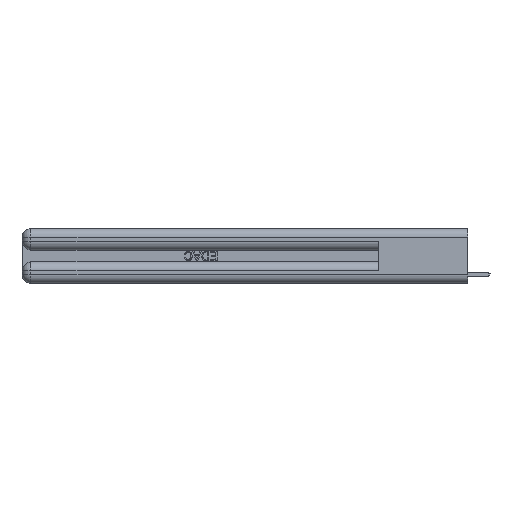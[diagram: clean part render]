
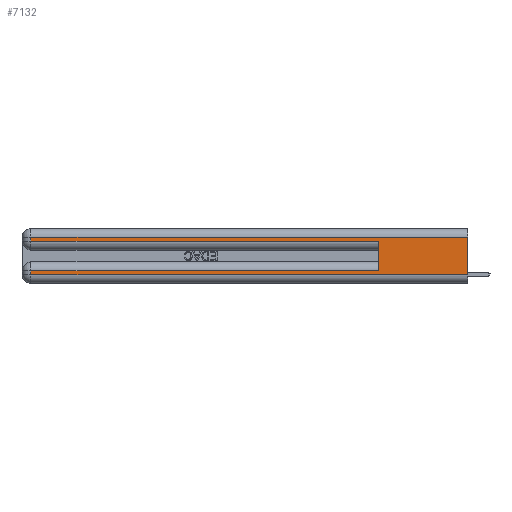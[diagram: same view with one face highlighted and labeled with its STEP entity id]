
A CAD part, left-side view. The second image highlights one B-rep face of the part: STEP entity #7132.
In plain terms, the highlighted planar face has unit normal (-1, 0, 0).
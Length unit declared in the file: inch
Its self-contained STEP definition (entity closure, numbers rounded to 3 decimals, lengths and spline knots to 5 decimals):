
#202 = VERTEX_POINT ( 'NONE', #26456 ) ;
#247 = ORIENTED_EDGE ( 'NONE', *, *, #23144, .T. ) ;
#1002 = LINE ( 'NONE', #12447, #19838 ) ;
#1217 = PLANE ( 'NONE',  #16699 ) ;
#1709 = DIRECTION ( 'NONE',  ( 0., 0., -1. ) ) ;
#1835 = VECTOR ( 'NONE', #1709, 39.37008 ) ;
#2278 = CARTESIAN_POINT ( 'NONE',  ( 0., 2.94, 0.285 ) ) ;
#2805 = VERTEX_POINT ( 'NONE', #8342 ) ;
#4398 = CARTESIAN_POINT ( 'NONE',  ( 0., 2.94, 0.31 ) ) ;
#4848 = VERTEX_POINT ( 'NONE', #4398 ) ;
#5518 = DIRECTION ( 'NONE',  ( 0., 0., 1. ) ) ;
#7132 = ADVANCED_FACE ( 'NONE', ( #8179 ), #1217, .F. ) ;
#7318 = ORIENTED_EDGE ( 'NONE', *, *, #28439, .F. ) ;
#7331 = VERTEX_POINT ( 'NONE', #2278 ) ;
#7342 = VECTOR ( 'NONE', #25105, 39.37008 ) ;
#8179 = FACE_OUTER_BOUND ( 'NONE', #25670, .T. ) ;
#8331 = EDGE_CURVE ( 'NONE', #16795, #16917, #10041, .T. ) ;
#8342 = CARTESIAN_POINT ( 'NONE',  ( 0., 2.94, 0.085 ) ) ;
#8874 = DIRECTION ( 'NONE',  ( 0., 0., -1. ) ) ;
#9269 = LINE ( 'NONE', #23933, #17684 ) ;
#10041 = LINE ( 'NONE', #17558, #7342 ) ;
#10042 = DIRECTION ( 'NONE',  ( 0., 1., 0. ) ) ;
#10367 = ORIENTED_EDGE ( 'NONE', *, *, #12968, .T. ) ;
#11068 = EDGE_CURVE ( 'NONE', #16795, #4848, #24806, .T. ) ;
#11350 = CARTESIAN_POINT ( 'NONE',  ( 0., 0., 0.37 ) ) ;
#11597 = ORIENTED_EDGE ( 'NONE', *, *, #25693, .T. ) ;
#12360 = VECTOR ( 'NONE', #14218, 39.37008 ) ;
#12447 = CARTESIAN_POINT ( 'NONE',  ( 0., 0.6, 0.145 ) ) ;
#12758 = LINE ( 'NONE', #21621, #12360 ) ;
#12968 = EDGE_CURVE ( 'NONE', #28253, #2805, #25993, .T. ) ;
#13055 = EDGE_CURVE ( 'NONE', #2805, #202, #27916, .T. ) ;
#13707 = CARTESIAN_POINT ( 'NONE',  ( 0., 2.94, 0.37 ) ) ;
#14218 = DIRECTION ( 'NONE',  ( 0., -1., 0. ) ) ;
#15268 = VECTOR ( 'NONE', #31707, 39.37008 ) ;
#15281 = CARTESIAN_POINT ( 'NONE',  ( 0., 0., 0.085 ) ) ;
#15297 = VECTOR ( 'NONE', #10042, 39.37008 ) ;
#16358 = CARTESIAN_POINT ( 'NONE',  ( 0., 2.94, 0.37 ) ) ;
#16699 = AXIS2_PLACEMENT_3D ( 'NONE', #11350, #28328, #8874 ) ;
#16795 = VERTEX_POINT ( 'NONE', #27718 ) ;
#16917 = VERTEX_POINT ( 'NONE', #21449 ) ;
#17558 = CARTESIAN_POINT ( 'NONE',  ( 0., 0., 0.37 ) ) ;
#17684 = VECTOR ( 'NONE', #24455, 39.37008 ) ;
#18268 = ORIENTED_EDGE ( 'NONE', *, *, #8331, .F. ) ;
#19838 = VECTOR ( 'NONE', #5518, 39.37008 ) ;
#21449 = CARTESIAN_POINT ( 'NONE',  ( 0., 0., 0.06 ) ) ;
#21621 = CARTESIAN_POINT ( 'NONE',  ( 0., 0., 0.06 ) ) ;
#22887 = VECTOR ( 'NONE', #25751, 39.37008 ) ;
#23090 = ORIENTED_EDGE ( 'NONE', *, *, #11068, .T. ) ;
#23144 = EDGE_CURVE ( 'NONE', #4848, #7331, #31331, .T. ) ;
#23933 = CARTESIAN_POINT ( 'NONE',  ( 0., 0., 0.285 ) ) ;
#24455 = DIRECTION ( 'NONE',  ( 0., -1., 0. ) ) ;
#24806 = LINE ( 'NONE', #26986, #15268 ) ;
#25105 = DIRECTION ( 'NONE',  ( 0., 0., -1. ) ) ;
#25608 = EDGE_CURVE ( 'NONE', #202, #16917, #12758, .T. ) ;
#25670 = EDGE_LOOP ( 'NONE', ( #18268, #23090, #247, #11597, #7318, #10367, #30464, #30754 ) ) ;
#25693 = EDGE_CURVE ( 'NONE', #7331, #28440, #9269, .T. ) ;
#25751 = DIRECTION ( 'NONE',  ( 0., 0., -1. ) ) ;
#25993 = LINE ( 'NONE', #15281, #15297 ) ;
#26456 = CARTESIAN_POINT ( 'NONE',  ( 0., 2.94, 0.06 ) ) ;
#26986 = CARTESIAN_POINT ( 'NONE',  ( 0., 0., 0.31 ) ) ;
#27718 = CARTESIAN_POINT ( 'NONE',  ( 0., 0., 0.31 ) ) ;
#27916 = LINE ( 'NONE', #16358, #1835 ) ;
#28253 = VERTEX_POINT ( 'NONE', #31584 ) ;
#28328 = DIRECTION ( 'NONE',  ( 1., 0., 0. ) ) ;
#28439 = EDGE_CURVE ( 'NONE', #28253, #28440, #1002, .T. ) ;
#28440 = VERTEX_POINT ( 'NONE', #29967 ) ;
#29967 = CARTESIAN_POINT ( 'NONE',  ( 0., 0.6, 0.285 ) ) ;
#30464 = ORIENTED_EDGE ( 'NONE', *, *, #13055, .T. ) ;
#30754 = ORIENTED_EDGE ( 'NONE', *, *, #25608, .T. ) ;
#31331 = LINE ( 'NONE', #13707, #22887 ) ;
#31584 = CARTESIAN_POINT ( 'NONE',  ( 0., 0.6, 0.085 ) ) ;
#31707 = DIRECTION ( 'NONE',  ( 0., 1., 0. ) ) ;
